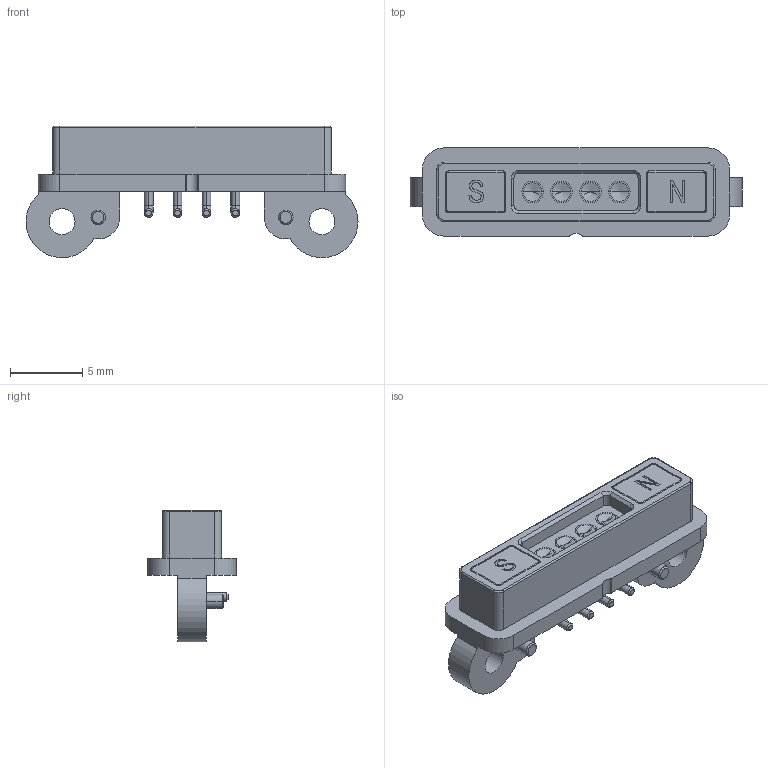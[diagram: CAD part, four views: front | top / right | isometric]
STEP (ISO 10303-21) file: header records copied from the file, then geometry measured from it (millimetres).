
FILE_DESCRIPTION (( 'STEP AP203' ), '1' );
FILE_NAME ('686-J0421350124.STEP', '2023-03-01T09:51:23', ( 'Magnum' ), ( '' ), 'SwSTEP 2.0', 'SolidWorks 2020', '' );
FILE_SCHEMA (( 'CONFIG_CONTROL_DESIGN' ));
Length unit declared in the file: millimetre
Products named in the file (1): 686-J0421350124
Bounding box: 23 x 6.1 x 9.09 mm (x, y, z)
Volume: 447.1 mm3; surface area: 778.9 mm2
Topology: 5 solids, 7 shells, 270 faces, 631 edges, 392 vertices
Faces by surface type: cylinder 104, plane 98, bspline 28, cone 26, torus 14
Entity records: 8640 total; most frequent: CARTESIAN_POINT 2378, DIRECTION 1327, ORIENTED_EDGE 1246, EDGE_CURVE 623, AXIS2_PLACEMENT_3D 501, VERTEX_POINT 392, VECTOR 325, LINE 325
